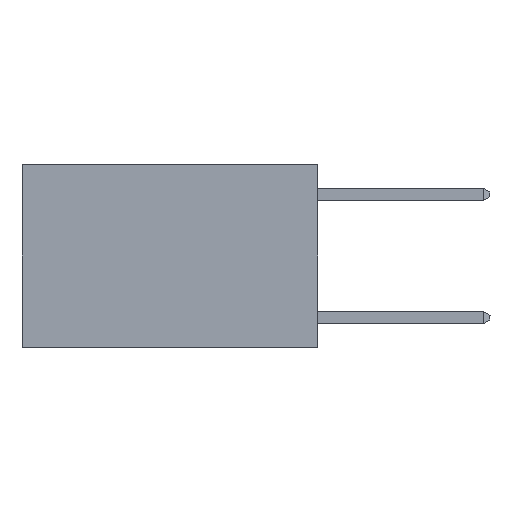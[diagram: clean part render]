
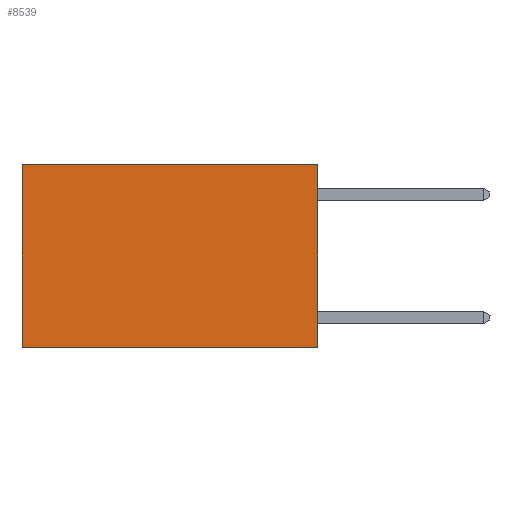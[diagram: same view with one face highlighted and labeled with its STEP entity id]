
A CAD part, left-side view. The second image highlights one B-rep face of the part: STEP entity #8539.
In plain terms, the highlighted planar face has unit normal (-1, 0, 0).
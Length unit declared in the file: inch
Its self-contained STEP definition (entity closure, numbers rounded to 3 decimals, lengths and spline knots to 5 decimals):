
#33 = VERTEX_POINT ( 'NONE', #24848 ) ;
#237 = CARTESIAN_POINT ( 'NONE',  ( 0.2625, 0.6, -0.37 ) ) ;
#1586 = VECTOR ( 'NONE', #25814, 39.37008 ) ;
#1613 = CARTESIAN_POINT ( 'NONE',  ( 0.2625, 0., -0.37 ) ) ;
#1664 = LINE ( 'NONE', #4441, #23796 ) ;
#3309 = EDGE_CURVE ( 'NONE', #33, #22864, #23830, .T. ) ;
#3565 = VERTEX_POINT ( 'NONE', #237 ) ;
#4411 = VECTOR ( 'NONE', #4544, 39.37008 ) ;
#4441 = CARTESIAN_POINT ( 'NONE',  ( 0.2625, 0., 0. ) ) ;
#4544 = DIRECTION ( 'NONE',  ( 0., 0., -1. ) ) ;
#5728 = CARTESIAN_POINT ( 'NONE',  ( 0.2625, 0., 0. ) ) ;
#5818 = DIRECTION ( 'NONE',  ( 0., 0., -1. ) ) ;
#7045 = LINE ( 'NONE', #1613, #1586 ) ;
#8539 = ADVANCED_FACE ( 'NONE', ( #19748 ), #13940, .F. ) ;
#9863 = LINE ( 'NONE', #24734, #4411 ) ;
#10583 = EDGE_CURVE ( 'NONE', #11625, #3565, #9863, .T. ) ;
#10763 = CARTESIAN_POINT ( 'NONE',  ( 0.2625, 0., 0. ) ) ;
#10924 = ORIENTED_EDGE ( 'NONE', *, *, #3309, .F. ) ;
#11625 = VERTEX_POINT ( 'NONE', #25654 ) ;
#13301 = CARTESIAN_POINT ( 'NONE',  ( 0.2625, 0., -0.37 ) ) ;
#13694 = EDGE_CURVE ( 'NONE', #22864, #3565, #7045, .T. ) ;
#13940 = PLANE ( 'NONE',  #20892 ) ;
#16762 = ORIENTED_EDGE ( 'NONE', *, *, #10583, .T. ) ;
#17749 = ORIENTED_EDGE ( 'NONE', *, *, #13694, .F. ) ;
#17775 = EDGE_CURVE ( 'NONE', #33, #11625, #1664, .T. ) ;
#17816 = ORIENTED_EDGE ( 'NONE', *, *, #17775, .T. ) ;
#17961 = VECTOR ( 'NONE', #18414, 39.37008 ) ;
#18000 = DIRECTION ( 'NONE',  ( 1., 0., 0. ) ) ;
#18414 = DIRECTION ( 'NONE',  ( 0., 0., -1. ) ) ;
#19748 = FACE_OUTER_BOUND ( 'NONE', #23600, .T. ) ;
#20892 = AXIS2_PLACEMENT_3D ( 'NONE', #5728, #18000, #5818 ) ;
#22864 = VERTEX_POINT ( 'NONE', #13301 ) ;
#23600 = EDGE_LOOP ( 'NONE', ( #16762, #17749, #10924, #17816 ) ) ;
#23796 = VECTOR ( 'NONE', #24560, 39.37008 ) ;
#23830 = LINE ( 'NONE', #10763, #17961 ) ;
#24560 = DIRECTION ( 'NONE',  ( 0., 1., 0. ) ) ;
#24734 = CARTESIAN_POINT ( 'NONE',  ( 0.2625, 0.6, 0. ) ) ;
#24848 = CARTESIAN_POINT ( 'NONE',  ( 0.2625, 0., 0. ) ) ;
#25654 = CARTESIAN_POINT ( 'NONE',  ( 0.2625, 0.6, 0. ) ) ;
#25814 = DIRECTION ( 'NONE',  ( 0., 1., 0. ) ) ;
